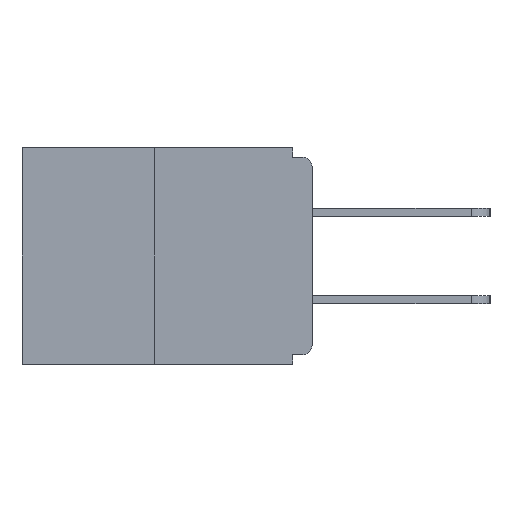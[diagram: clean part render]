
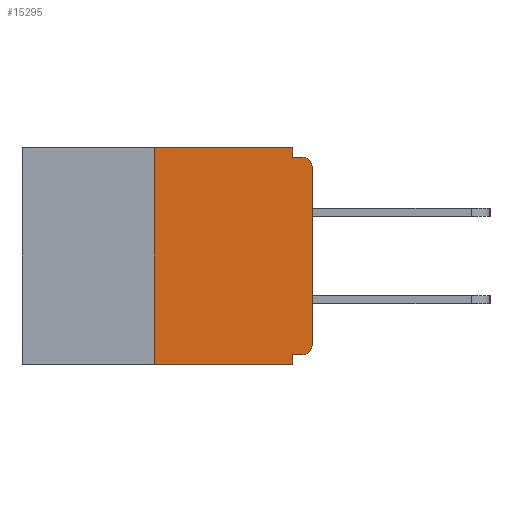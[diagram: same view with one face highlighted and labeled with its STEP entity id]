
A CAD part, left-side view. The second image highlights one B-rep face of the part: STEP entity #15295.
In plain terms, the highlighted planar face has unit normal (-1, 0, 0).
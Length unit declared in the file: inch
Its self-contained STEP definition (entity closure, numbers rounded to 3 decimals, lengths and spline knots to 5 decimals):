
#840 = ORIENTED_EDGE ( 'NONE', *, *, #14948, .T. ) ;
#1342 = VERTEX_POINT ( 'NONE', #17165 ) ;
#1436 = CIRCLE ( 'NONE', #16196, 0.015 ) ;
#1565 = DIRECTION ( 'NONE',  ( 0., 0., -1. ) ) ;
#1587 = DIRECTION ( 'NONE',  ( 0., 0., -1. ) ) ;
#1776 = VECTOR ( 'NONE', #12981, 39.37008 ) ;
#1799 = VERTEX_POINT ( 'NONE', #18290 ) ;
#2028 = ORIENTED_EDGE ( 'NONE', *, *, #3013, .F. ) ;
#2795 = EDGE_CURVE ( 'NONE', #16603, #1799, #7721, .T. ) ;
#2822 = EDGE_CURVE ( 'NONE', #15411, #22041, #15668, .T. ) ;
#2880 = DIRECTION ( 'NONE',  ( 0., -1., 0. ) ) ;
#2884 = ORIENTED_EDGE ( 'NONE', *, *, #8151, .T. ) ;
#2921 = DIRECTION ( 'NONE',  ( 0., 0., 1. ) ) ;
#3013 = EDGE_CURVE ( 'NONE', #19999, #16603, #3637, .T. ) ;
#3258 = VECTOR ( 'NONE', #2921, 39.37008 ) ;
#3626 = CARTESIAN_POINT ( 'NONE',  ( 0., 0.031, -0.343 ) ) ;
#3637 = LINE ( 'NONE', #8401, #23069 ) ;
#3727 = CARTESIAN_POINT ( 'NONE',  ( 0., 0.25, 0. ) ) ;
#3971 = CARTESIAN_POINT ( 'NONE',  ( 0., 0.015, -0.313 ) ) ;
#4331 = VERTEX_POINT ( 'NONE', #3727 ) ;
#4337 = ORIENTED_EDGE ( 'NONE', *, *, #24151, .F. ) ;
#4603 = ORIENTED_EDGE ( 'NONE', *, *, #16146, .F. ) ;
#5334 = DIRECTION ( 'NONE',  ( 1., 0., 0. ) ) ;
#5390 = DIRECTION ( 'NONE',  ( 0., 0., 1. ) ) ;
#5442 = DIRECTION ( 'NONE',  ( 0., -1., 0. ) ) ;
#5451 = CARTESIAN_POINT ( 'NONE',  ( 0., 0.46, -0.343 ) ) ;
#5869 = VERTEX_POINT ( 'NONE', #23320 ) ;
#5949 = DIRECTION ( 'NONE',  ( -1., 0., 0. ) ) ;
#7017 = ORIENTED_EDGE ( 'NONE', *, *, #13558, .T. ) ;
#7127 = DIRECTION ( 'NONE',  ( 0., 0., -1. ) ) ;
#7253 = DIRECTION ( 'NONE',  ( -1., 0., 0. ) ) ;
#7331 = ORIENTED_EDGE ( 'NONE', *, *, #2822, .F. ) ;
#7721 = LINE ( 'NONE', #12225, #18341 ) ;
#8100 = CARTESIAN_POINT ( 'NONE',  ( 0., 0., 0. ) ) ;
#8151 = EDGE_CURVE ( 'NONE', #20983, #1342, #18266, .T. ) ;
#8401 = CARTESIAN_POINT ( 'NONE',  ( 0., 0.031, 0. ) ) ;
#8988 = CARTESIAN_POINT ( 'NONE',  ( 0., 0.46, 0. ) ) ;
#9457 = EDGE_LOOP ( 'NONE', ( #11169, #4603, #2884, #4337, #7331, #840, #7017, #10921, #24061, #2028 ) ) ;
#9475 = VECTOR ( 'NONE', #22291, 39.37008 ) ;
#10824 = CARTESIAN_POINT ( 'NONE',  ( 0., 0.031, -0.015 ) ) ;
#10921 = ORIENTED_EDGE ( 'NONE', *, *, #11561, .T. ) ;
#11169 = ORIENTED_EDGE ( 'NONE', *, *, #18078, .F. ) ;
#11561 = EDGE_CURVE ( 'NONE', #16410, #1799, #22841, .T. ) ;
#11782 = LINE ( 'NONE', #8100, #3258 ) ;
#11857 = CARTESIAN_POINT ( 'NONE',  ( 0., 0.031, 0. ) ) ;
#12225 = CARTESIAN_POINT ( 'NONE',  ( 0., 0., -0.015 ) ) ;
#12854 = CARTESIAN_POINT ( 'NONE',  ( 0., 0.031, -0.328 ) ) ;
#12902 = CARTESIAN_POINT ( 'NONE',  ( 0., 0.015, -0.03 ) ) ;
#12981 = DIRECTION ( 'NONE',  ( 0., -1., 0. ) ) ;
#13145 = VECTOR ( 'NONE', #1565, 39.37008 ) ;
#13558 = EDGE_CURVE ( 'NONE', #5869, #16410, #11782, .T. ) ;
#13613 = DIRECTION ( 'NONE',  ( 0., 0., -1. ) ) ;
#14788 = VECTOR ( 'NONE', #5390, 39.37008 ) ;
#14948 = EDGE_CURVE ( 'NONE', #15411, #5869, #1436, .T. ) ;
#15082 = LINE ( 'NONE', #22261, #14788 ) ;
#15295 = ADVANCED_FACE ( 'NONE', ( #19132 ), #22209, .F. ) ;
#15411 = VERTEX_POINT ( 'NONE', #16421 ) ;
#15668 = LINE ( 'NONE', #18609, #9475 ) ;
#16146 = EDGE_CURVE ( 'NONE', #20983, #4331, #15082, .T. ) ;
#16196 = AXIS2_PLACEMENT_3D ( 'NONE', #3971, #5949, #13613 ) ;
#16410 = VERTEX_POINT ( 'NONE', #18278 ) ;
#16421 = CARTESIAN_POINT ( 'NONE',  ( 0., 0.015, -0.328 ) ) ;
#16603 = VERTEX_POINT ( 'NONE', #10824 ) ;
#16691 = AXIS2_PLACEMENT_3D ( 'NONE', #8988, #5334, #7127 ) ;
#17165 = CARTESIAN_POINT ( 'NONE',  ( 0., 0.031, -0.343 ) ) ;
#18078 = EDGE_CURVE ( 'NONE', #4331, #19999, #23305, .T. ) ;
#18266 = LINE ( 'NONE', #5451, #1776 ) ;
#18278 = CARTESIAN_POINT ( 'NONE',  ( 0., 0., -0.03 ) ) ;
#18290 = CARTESIAN_POINT ( 'NONE',  ( 0., 0.015, -0.015 ) ) ;
#18341 = VECTOR ( 'NONE', #2880, 39.37008 ) ;
#18552 = CARTESIAN_POINT ( 'NONE',  ( 0., 0.46, 0. ) ) ;
#18609 = CARTESIAN_POINT ( 'NONE',  ( 0., 0., -0.328 ) ) ;
#19132 = FACE_OUTER_BOUND ( 'NONE', #9457, .T. ) ;
#19981 = LINE ( 'NONE', #3626, #13145 ) ;
#19999 = VERTEX_POINT ( 'NONE', #11857 ) ;
#20983 = VERTEX_POINT ( 'NONE', #23391 ) ;
#21604 = DIRECTION ( 'NONE',  ( 0., 0., -1. ) ) ;
#22041 = VERTEX_POINT ( 'NONE', #12854 ) ;
#22192 = AXIS2_PLACEMENT_3D ( 'NONE', #12902, #7253, #1587 ) ;
#22209 = PLANE ( 'NONE',  #16691 ) ;
#22261 = CARTESIAN_POINT ( 'NONE',  ( 0., 0.25, 0. ) ) ;
#22291 = DIRECTION ( 'NONE',  ( 0., 1., 0. ) ) ;
#22841 = CIRCLE ( 'NONE', #22192, 0.015 ) ;
#23069 = VECTOR ( 'NONE', #21604, 39.37008 ) ;
#23305 = LINE ( 'NONE', #18552, #23899 ) ;
#23320 = CARTESIAN_POINT ( 'NONE',  ( 0., 0., -0.313 ) ) ;
#23391 = CARTESIAN_POINT ( 'NONE',  ( 0., 0.25, -0.343 ) ) ;
#23899 = VECTOR ( 'NONE', #5442, 39.37008 ) ;
#24061 = ORIENTED_EDGE ( 'NONE', *, *, #2795, .F. ) ;
#24151 = EDGE_CURVE ( 'NONE', #22041, #1342, #19981, .T. ) ;
